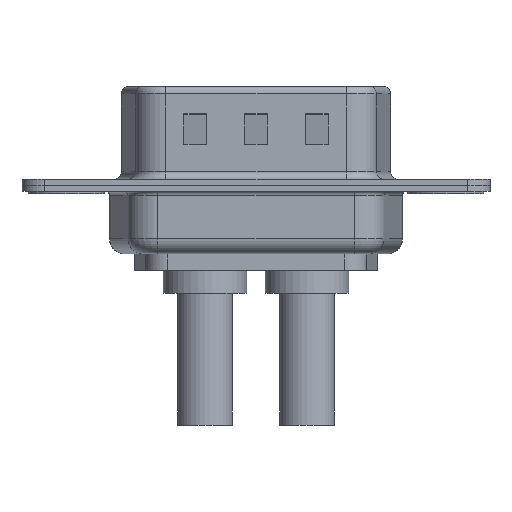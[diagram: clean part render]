
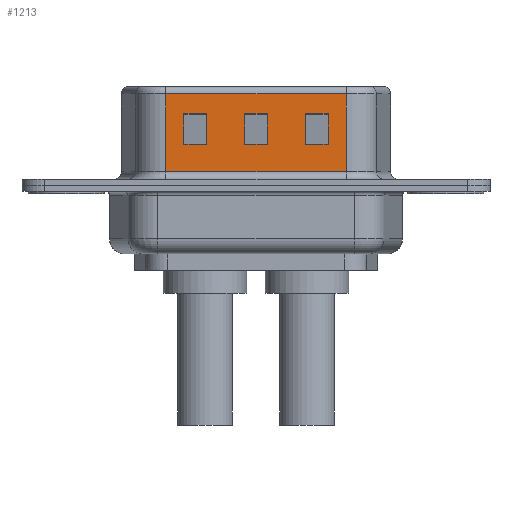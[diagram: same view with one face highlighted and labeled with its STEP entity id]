
A CAD part, front view. The second image highlights one B-rep face of the part: STEP entity #1213.
In plain terms, the highlighted planar face has unit normal (0, -1, 0).
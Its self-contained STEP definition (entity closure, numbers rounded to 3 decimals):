
#35 = ORIENTED_EDGE ( 'NONE', *, *, #3612, .T. ) ;
#109 = ORIENTED_EDGE ( 'NONE', *, *, #7643, .T. ) ;
#140 = ORIENTED_EDGE ( 'NONE', *, *, #4446, .T. ) ;
#252 = ORIENTED_EDGE ( 'NONE', *, *, #12139, .T. ) ;
#338 = LINE ( 'NONE', #7841, #7970 ) ;
#360 = CARTESIAN_POINT ( 'NONE',  ( 18.45, -4.58, 6.52 ) ) ;
#622 = CARTESIAN_POINT ( 'NONE',  ( 18.45, -4.58, 0.9 ) ) ;
#670 = LINE ( 'NONE', #3397, #8230 ) ;
#753 = AXIS2_PLACEMENT_3D ( 'NONE', #360, #11141, #3674 ) ;
#1020 = EDGE_CURVE ( 'NONE', #10791, #5941, #8758, .T. ) ;
#1074 = VECTOR ( 'NONE', #5228, 1000. ) ;
#1104 = VECTOR ( 'NONE', #9176, 1000. ) ;
#1119 = VECTOR ( 'NONE', #6582, 1000. ) ;
#1213 = ADVANCED_FACE ( 'NONE', ( #6905, #1589, #2229, #4238 ), #2258, .F. ) ;
#1395 = VERTEX_POINT ( 'NONE', #4732 ) ;
#1431 = VECTOR ( 'NONE', #3999, 1000. ) ;
#1515 = EDGE_CURVE ( 'NONE', #1395, #7785, #8746, .T. ) ;
#1589 = FACE_BOUND ( 'NONE', #4599, .T. ) ;
#1865 = EDGE_CURVE ( 'NONE', #3654, #4944, #11518, .T. ) ;
#1943 = EDGE_CURVE ( 'NONE', #3297, #3654, #10245, .T. ) ;
#2053 = VECTOR ( 'NONE', #5812, 1000. ) ;
#2218 = LINE ( 'NONE', #8512, #4555 ) ;
#2229 = FACE_BOUND ( 'NONE', #5768, .T. ) ;
#2258 = PLANE ( 'NONE',  #753 ) ;
#2300 = CARTESIAN_POINT ( 'NONE',  ( 7.75, -4.58, 4.705 ) ) ;
#2427 = VERTEX_POINT ( 'NONE', #3171 ) ;
#2437 = CARTESIAN_POINT ( 'NONE',  ( 14.45, -4.58, 4.705 ) ) ;
#2698 = CARTESIAN_POINT ( 'NONE',  ( 22.45, -4.58, 4.705 ) ) ;
#2788 = EDGE_CURVE ( 'NONE', #7785, #3451, #7981, .T. ) ;
#2864 = DIRECTION ( 'NONE',  ( 0., 0., -1. ) ) ;
#2912 = VERTEX_POINT ( 'NONE', #11422 ) ;
#3040 = ORIENTED_EDGE ( 'NONE', *, *, #1865, .T. ) ;
#3079 = VERTEX_POINT ( 'NONE', #11464 ) ;
#3154 = DIRECTION ( 'NONE',  ( -1., 0., 0. ) ) ;
#3171 = CARTESIAN_POINT ( 'NONE',  ( 11.75, -4.58, 2.705 ) ) ;
#3239 = LINE ( 'NONE', #5799, #7955 ) ;
#3265 = VECTOR ( 'NONE', #4658, 1000. ) ;
#3297 = VERTEX_POINT ( 'NONE', #6641 ) ;
#3397 = CARTESIAN_POINT ( 'NONE',  ( 18.45, -4.58, 2.705 ) ) ;
#3451 = VERTEX_POINT ( 'NONE', #2300 ) ;
#3565 = CARTESIAN_POINT ( 'NONE',  ( 18.45, -4.58, 6.02 ) ) ;
#3612 = EDGE_CURVE ( 'NONE', #2912, #1395, #8547, .T. ) ;
#3654 = VERTEX_POINT ( 'NONE', #8952 ) ;
#3674 = DIRECTION ( 'NONE',  ( 0., 0., 1. ) ) ;
#3814 = ORIENTED_EDGE ( 'NONE', *, *, #5415, .T. ) ;
#3821 = DIRECTION ( 'NONE',  ( 0., 0., -1. ) ) ;
#3885 = DIRECTION ( 'NONE',  ( 0., 0., 1. ) ) ;
#3983 = CARTESIAN_POINT ( 'NONE',  ( 7.75, -4.58, 6.52 ) ) ;
#3999 = DIRECTION ( 'NONE',  ( -1., 0., 0. ) ) ;
#4053 = ORIENTED_EDGE ( 'NONE', *, *, #2788, .T. ) ;
#4161 = DIRECTION ( 'NONE',  ( 1., 0., 0. ) ) ;
#4195 = CARTESIAN_POINT ( 'NONE',  ( 11.75, -4.58, 4.705 ) ) ;
#4238 = FACE_OUTER_BOUND ( 'NONE', #12442, .T. ) ;
#4261 = CARTESIAN_POINT ( 'NONE',  ( 18.45, -4.58, 6.02 ) ) ;
#4446 = EDGE_CURVE ( 'NONE', #2427, #11733, #9842, .T. ) ;
#4484 = ORIENTED_EDGE ( 'NONE', *, *, #12316, .T. ) ;
#4555 = VECTOR ( 'NONE', #2864, 1000. ) ;
#4583 = VERTEX_POINT ( 'NONE', #5700 ) ;
#4599 = EDGE_LOOP ( 'NONE', ( #4917, #6264, #3040, #109 ) ) ;
#4658 = DIRECTION ( 'NONE',  ( 0., 0., -1. ) ) ;
#4732 = CARTESIAN_POINT ( 'NONE',  ( 9.25, -4.58, 2.705 ) ) ;
#4787 = LINE ( 'NONE', #8135, #6817 ) ;
#4917 = ORIENTED_EDGE ( 'NONE', *, *, #12612, .T. ) ;
#4944 = VERTEX_POINT ( 'NONE', #9034 ) ;
#5111 = DIRECTION ( 'NONE',  ( 1., 0., 0. ) ) ;
#5201 = ORIENTED_EDGE ( 'NONE', *, *, #8586, .F. ) ;
#5228 = DIRECTION ( 'NONE',  ( 1., 0., 0. ) ) ;
#5363 = VERTEX_POINT ( 'NONE', #622 ) ;
#5415 = EDGE_CURVE ( 'NONE', #3451, #2912, #9683, .T. ) ;
#5631 = VERTEX_POINT ( 'NONE', #9723 ) ;
#5700 = CARTESIAN_POINT ( 'NONE',  ( 13.25, -4.58, 2.705 ) ) ;
#5768 = EDGE_LOOP ( 'NONE', ( #4484, #252, #7449, #140 ) ) ;
#5799 = CARTESIAN_POINT ( 'NONE',  ( 17.25, -4.58, 6.52 ) ) ;
#5805 = EDGE_LOOP ( 'NONE', ( #35, #6471, #4053, #3814 ) ) ;
#5812 = DIRECTION ( 'NONE',  ( -1., 0., 0. ) ) ;
#5941 = VERTEX_POINT ( 'NONE', #9840 ) ;
#6114 = CARTESIAN_POINT ( 'NONE',  ( 15.75, -4.58, 6.52 ) ) ;
#6264 = ORIENTED_EDGE ( 'NONE', *, *, #1943, .T. ) ;
#6304 = LINE ( 'NONE', #2698, #8254 ) ;
#6453 = LINE ( 'NONE', #9209, #1104 ) ;
#6471 = ORIENTED_EDGE ( 'NONE', *, *, #1515, .T. ) ;
#6582 = DIRECTION ( 'NONE',  ( -1., 0., 0. ) ) ;
#6641 = CARTESIAN_POINT ( 'NONE',  ( 17.25, -4.58, 2.705 ) ) ;
#6719 = VERTEX_POINT ( 'NONE', #9173 ) ;
#6817 = VECTOR ( 'NONE', #4161, 1000. ) ;
#6832 = EDGE_CURVE ( 'NONE', #5941, #3079, #2218, .T. ) ;
#6886 = CARTESIAN_POINT ( 'NONE',  ( 11.75, -4.58, 6.52 ) ) ;
#6905 = FACE_BOUND ( 'NONE', #5805, .T. ) ;
#7240 = VECTOR ( 'NONE', #9549, 1000. ) ;
#7322 = VECTOR ( 'NONE', #3885, 1000. ) ;
#7449 = ORIENTED_EDGE ( 'NONE', *, *, #9364, .T. ) ;
#7601 = ORIENTED_EDGE ( 'NONE', *, *, #1020, .T. ) ;
#7643 = EDGE_CURVE ( 'NONE', #4944, #5631, #6304, .T. ) ;
#7785 = VERTEX_POINT ( 'NONE', #9646 ) ;
#7841 = CARTESIAN_POINT ( 'NONE',  ( 13.25, -4.58, 6.52 ) ) ;
#7955 = VECTOR ( 'NONE', #12690, 1000. ) ;
#7970 = VECTOR ( 'NONE', #3821, 1000. ) ;
#7981 = LINE ( 'NONE', #3983, #7322 ) ;
#8135 = CARTESIAN_POINT ( 'NONE',  ( 18.45, -4.58, 0.9 ) ) ;
#8230 = VECTOR ( 'NONE', #3154, 1000. ) ;
#8254 = VECTOR ( 'NONE', #12352, 1000. ) ;
#8512 = CARTESIAN_POINT ( 'NONE',  ( 6.55, -4.58, 6.52 ) ) ;
#8547 = LINE ( 'NONE', #10983, #3265 ) ;
#8586 = EDGE_CURVE ( 'NONE', #10791, #5363, #6453, .T. ) ;
#8746 = LINE ( 'NONE', #12276, #1119 ) ;
#8758 = LINE ( 'NONE', #3565, #1431 ) ;
#8952 = CARTESIAN_POINT ( 'NONE',  ( 15.75, -4.58, 2.705 ) ) ;
#9034 = CARTESIAN_POINT ( 'NONE',  ( 15.75, -4.58, 4.705 ) ) ;
#9173 = CARTESIAN_POINT ( 'NONE',  ( 13.25, -4.58, 4.705 ) ) ;
#9176 = DIRECTION ( 'NONE',  ( 0., 0., -1. ) ) ;
#9209 = CARTESIAN_POINT ( 'NONE',  ( 18.45, -4.58, 6.52 ) ) ;
#9364 = EDGE_CURVE ( 'NONE', #4583, #2427, #670, .T. ) ;
#9549 = DIRECTION ( 'NONE',  ( 0., 0., 1. ) ) ;
#9646 = CARTESIAN_POINT ( 'NONE',  ( 7.75, -4.58, 2.705 ) ) ;
#9683 = LINE ( 'NONE', #2437, #11384 ) ;
#9723 = CARTESIAN_POINT ( 'NONE',  ( 17.25, -4.58, 4.705 ) ) ;
#9840 = CARTESIAN_POINT ( 'NONE',  ( 6.55, -4.58, 6.02 ) ) ;
#9842 = LINE ( 'NONE', #6886, #7240 ) ;
#10245 = LINE ( 'NONE', #11205, #2053 ) ;
#10417 = ORIENTED_EDGE ( 'NONE', *, *, #11218, .T. ) ;
#10568 = VECTOR ( 'NONE', #10605, 1000. ) ;
#10605 = DIRECTION ( 'NONE',  ( 0., 0., 1. ) ) ;
#10791 = VERTEX_POINT ( 'NONE', #4261 ) ;
#10983 = CARTESIAN_POINT ( 'NONE',  ( 9.25, -4.58, 6.52 ) ) ;
#11141 = DIRECTION ( 'NONE',  ( 0., 1., 0. ) ) ;
#11205 = CARTESIAN_POINT ( 'NONE',  ( 22.45, -4.58, 2.705 ) ) ;
#11218 = EDGE_CURVE ( 'NONE', #3079, #5363, #4787, .T. ) ;
#11304 = LINE ( 'NONE', #12103, #1074 ) ;
#11384 = VECTOR ( 'NONE', #5111, 1000. ) ;
#11422 = CARTESIAN_POINT ( 'NONE',  ( 9.25, -4.58, 4.705 ) ) ;
#11464 = CARTESIAN_POINT ( 'NONE',  ( 6.55, -4.58, 0.9 ) ) ;
#11518 = LINE ( 'NONE', #6114, #10568 ) ;
#11733 = VERTEX_POINT ( 'NONE', #4195 ) ;
#12103 = CARTESIAN_POINT ( 'NONE',  ( 18.45, -4.58, 4.705 ) ) ;
#12139 = EDGE_CURVE ( 'NONE', #6719, #4583, #338, .T. ) ;
#12276 = CARTESIAN_POINT ( 'NONE',  ( 14.45, -4.58, 2.705 ) ) ;
#12316 = EDGE_CURVE ( 'NONE', #11733, #6719, #11304, .T. ) ;
#12352 = DIRECTION ( 'NONE',  ( 1., 0., 0. ) ) ;
#12442 = EDGE_LOOP ( 'NONE', ( #5201, #7601, #12686, #10417 ) ) ;
#12612 = EDGE_CURVE ( 'NONE', #5631, #3297, #3239, .T. ) ;
#12686 = ORIENTED_EDGE ( 'NONE', *, *, #6832, .T. ) ;
#12690 = DIRECTION ( 'NONE',  ( 0., 0., -1. ) ) ;
